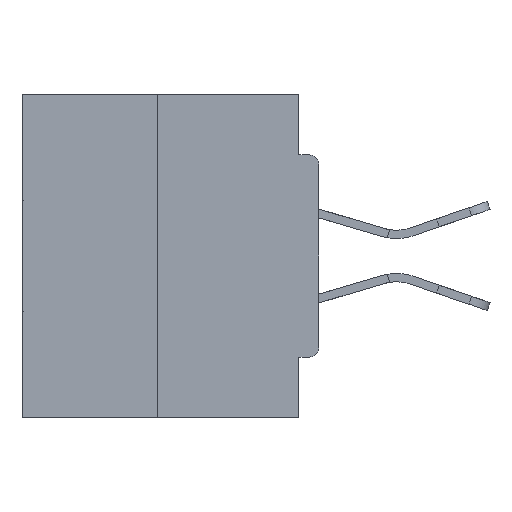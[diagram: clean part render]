
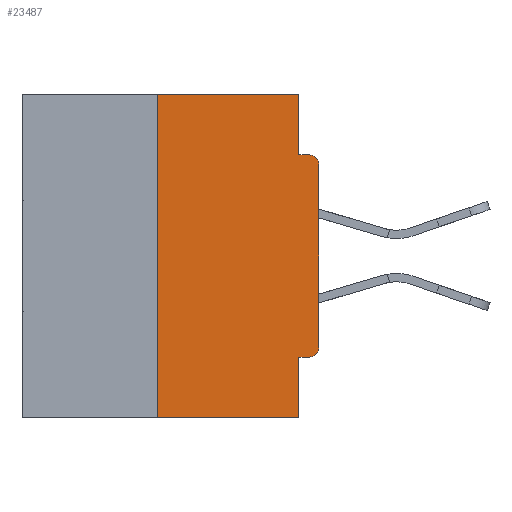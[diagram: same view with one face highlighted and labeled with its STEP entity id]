
A CAD part, left-side view. The second image highlights one B-rep face of the part: STEP entity #23487.
In plain terms, the highlighted planar face has unit normal (-1, 0, 0).
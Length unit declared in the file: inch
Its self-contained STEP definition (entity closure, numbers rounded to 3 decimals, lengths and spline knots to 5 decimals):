
#166 = LINE ( 'NONE', #5510, #31849 ) ;
#188 = DIRECTION ( 'NONE',  ( 0., 0., 1. ) ) ;
#624 = CARTESIAN_POINT ( 'NONE',  ( 0., 0.031, -0.0935 ) ) ;
#775 = CARTESIAN_POINT ( 'NONE',  ( 0., 0.25, 0. ) ) ;
#1458 = DIRECTION ( 'NONE',  ( 0., 0., -1. ) ) ;
#1505 = EDGE_CURVE ( 'NONE', #5066, #21677, #22919, .T. ) ;
#1512 = ORIENTED_EDGE ( 'NONE', *, *, #37191, .F. ) ;
#1676 = CARTESIAN_POINT ( 'NONE',  ( 0., 0., -0.3915 ) ) ;
#2341 = VERTEX_POINT ( 'NONE', #19282 ) ;
#2542 = ORIENTED_EDGE ( 'NONE', *, *, #22281, .T. ) ;
#2605 = EDGE_CURVE ( 'NONE', #20122, #21006, #23744, .T. ) ;
#2826 = LINE ( 'NONE', #6681, #20943 ) ;
#2867 = ORIENTED_EDGE ( 'NONE', *, *, #2605, .T. ) ;
#3800 = VECTOR ( 'NONE', #37121, 39.37008 ) ;
#3911 = DIRECTION ( 'NONE',  ( 0., 1., 0. ) ) ;
#5066 = VERTEX_POINT ( 'NONE', #13340 ) ;
#5510 = CARTESIAN_POINT ( 'NONE',  ( 0., 0.031, -0.5 ) ) ;
#5576 = CARTESIAN_POINT ( 'NONE',  ( 0., 0.031, -0.4065 ) ) ;
#5696 = FACE_OUTER_BOUND ( 'NONE', #8091, .T. ) ;
#5751 = ORIENTED_EDGE ( 'NONE', *, *, #13193, .F. ) ;
#5893 = DIRECTION ( 'NONE',  ( 0., -1., 0. ) ) ;
#6483 = DIRECTION ( 'NONE',  ( 0., 0., -1. ) ) ;
#6681 = CARTESIAN_POINT ( 'NONE',  ( 0., 0., -0.4065 ) ) ;
#7240 = LINE ( 'NONE', #775, #30833 ) ;
#7283 = DIRECTION ( 'NONE',  ( 1., 0., 0. ) ) ;
#7732 = VECTOR ( 'NONE', #188, 39.37008 ) ;
#8091 = EDGE_LOOP ( 'NONE', ( #1512, #12198, #20064, #5751, #32078, #2867, #22554, #2542, #9001, #38771 ) ) ;
#8362 = EDGE_CURVE ( 'NONE', #32576, #2341, #7240, .T. ) ;
#8741 = EDGE_CURVE ( 'NONE', #21677, #17403, #37108, .T. ) ;
#9001 = ORIENTED_EDGE ( 'NONE', *, *, #8741, .F. ) ;
#9575 = DIRECTION ( 'NONE',  ( -1., 0., 0. ) ) ;
#9688 = VERTEX_POINT ( 'NONE', #24381 ) ;
#11065 = AXIS2_PLACEMENT_3D ( 'NONE', #11961, #13028, #6483 ) ;
#11961 = CARTESIAN_POINT ( 'NONE',  ( 0., 0.015, -0.3915 ) ) ;
#12057 = CARTESIAN_POINT ( 'NONE',  ( 0., 0., 0. ) ) ;
#12198 = ORIENTED_EDGE ( 'NONE', *, *, #8362, .F. ) ;
#12430 = EDGE_CURVE ( 'NONE', #21006, #22560, #27911, .T. ) ;
#12664 = CARTESIAN_POINT ( 'NONE',  ( 0., 0.015, -0.1085 ) ) ;
#13028 = DIRECTION ( 'NONE',  ( -1., 0., 0. ) ) ;
#13193 = EDGE_CURVE ( 'NONE', #28718, #9688, #166, .T. ) ;
#13340 = CARTESIAN_POINT ( 'NONE',  ( 0., 0.031, 0. ) ) ;
#13421 = DIRECTION ( 'NONE',  ( 0., 0., 1. ) ) ;
#14013 = CARTESIAN_POINT ( 'NONE',  ( 0., 0., -0.1085 ) ) ;
#17403 = VERTEX_POINT ( 'NONE', #35831 ) ;
#18924 = VECTOR ( 'NONE', #34775, 39.37008 ) ;
#19282 = CARTESIAN_POINT ( 'NONE',  ( 0., 0.25, 0. ) ) ;
#19363 = CARTESIAN_POINT ( 'NONE',  ( 0., 0.46, 0. ) ) ;
#19855 = CIRCLE ( 'NONE', #36661, 0.015 ) ;
#20064 = ORIENTED_EDGE ( 'NONE', *, *, #23283, .T. ) ;
#20122 = VERTEX_POINT ( 'NONE', #25848 ) ;
#20282 = CARTESIAN_POINT ( 'NONE',  ( 0., 0.46, -0.5 ) ) ;
#20943 = VECTOR ( 'NONE', #3911, 39.37008 ) ;
#21006 = VERTEX_POINT ( 'NONE', #1676 ) ;
#21568 = VECTOR ( 'NONE', #5893, 39.37008 ) ;
#21677 = VERTEX_POINT ( 'NONE', #624 ) ;
#21909 = VECTOR ( 'NONE', #27019, 39.37008 ) ;
#22281 = EDGE_CURVE ( 'NONE', #22560, #17403, #19855, .T. ) ;
#22403 = AXIS2_PLACEMENT_3D ( 'NONE', #19363, #7283, #1458 ) ;
#22554 = ORIENTED_EDGE ( 'NONE', *, *, #12430, .T. ) ;
#22560 = VERTEX_POINT ( 'NONE', #14013 ) ;
#22919 = LINE ( 'NONE', #36838, #3800 ) ;
#23113 = EDGE_CURVE ( 'NONE', #20122, #28718, #2826, .T. ) ;
#23283 = EDGE_CURVE ( 'NONE', #32576, #9688, #26217, .T. ) ;
#23487 = ADVANCED_FACE ( 'NONE', ( #5696 ), #37895, .F. ) ;
#23744 = CIRCLE ( 'NONE', #11065, 0.015 ) ;
#24183 = LINE ( 'NONE', #28238, #18924 ) ;
#24381 = CARTESIAN_POINT ( 'NONE',  ( 0., 0.031, -0.5 ) ) ;
#25848 = CARTESIAN_POINT ( 'NONE',  ( 0., 0.015, -0.4065 ) ) ;
#26217 = LINE ( 'NONE', #20282, #21909 ) ;
#27019 = DIRECTION ( 'NONE',  ( 0., -1., 0. ) ) ;
#27911 = LINE ( 'NONE', #12057, #7732 ) ;
#28238 = CARTESIAN_POINT ( 'NONE',  ( 0., 0.46, 0. ) ) ;
#28718 = VERTEX_POINT ( 'NONE', #5576 ) ;
#29165 = CARTESIAN_POINT ( 'NONE',  ( 0., 0.25, -0.5 ) ) ;
#30833 = VECTOR ( 'NONE', #13421, 39.37008 ) ;
#31389 = DIRECTION ( 'NONE',  ( 0., 0., -1. ) ) ;
#31849 = VECTOR ( 'NONE', #39673, 39.37008 ) ;
#32078 = ORIENTED_EDGE ( 'NONE', *, *, #23113, .F. ) ;
#32576 = VERTEX_POINT ( 'NONE', #29165 ) ;
#33585 = CARTESIAN_POINT ( 'NONE',  ( 0., 0., -0.0935 ) ) ;
#34775 = DIRECTION ( 'NONE',  ( 0., -1., 0. ) ) ;
#35831 = CARTESIAN_POINT ( 'NONE',  ( 0., 0.015, -0.0935 ) ) ;
#36661 = AXIS2_PLACEMENT_3D ( 'NONE', #12664, #9575, #31389 ) ;
#36838 = CARTESIAN_POINT ( 'NONE',  ( 0., 0.031, 0. ) ) ;
#37108 = LINE ( 'NONE', #33585, #21568 ) ;
#37121 = DIRECTION ( 'NONE',  ( 0., 0., -1. ) ) ;
#37191 = EDGE_CURVE ( 'NONE', #2341, #5066, #24183, .T. ) ;
#37895 = PLANE ( 'NONE',  #22403 ) ;
#38771 = ORIENTED_EDGE ( 'NONE', *, *, #1505, .F. ) ;
#39673 = DIRECTION ( 'NONE',  ( 0., 0., -1. ) ) ;
